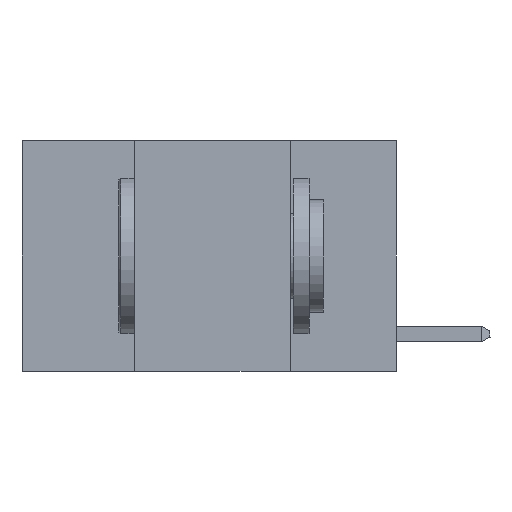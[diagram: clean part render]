
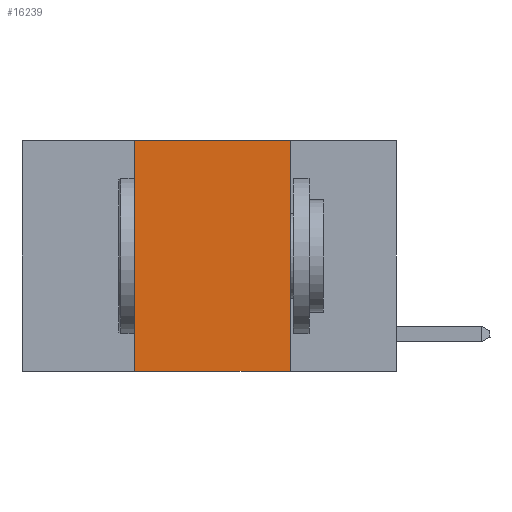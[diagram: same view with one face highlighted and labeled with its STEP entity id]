
A CAD part, left-side view. The second image highlights one B-rep face of the part: STEP entity #16239.
In plain terms, the highlighted planar face has unit normal (-1, 0, 0).
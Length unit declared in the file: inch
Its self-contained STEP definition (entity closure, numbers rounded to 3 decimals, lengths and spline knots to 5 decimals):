
#357 = VECTOR ( 'NONE', #3795, 39.37008 ) ;
#949 = VECTOR ( 'NONE', #24811, 39.37008 ) ;
#987 = DIRECTION ( 'NONE',  ( 0., -1., 0. ) ) ;
#1590 = CARTESIAN_POINT ( 'NONE',  ( 0., 0.17, 0. ) ) ;
#3172 = ORIENTED_EDGE ( 'NONE', *, *, #14653, .F. ) ;
#3487 = DIRECTION ( 'NONE',  ( 0., 0., 1. ) ) ;
#3795 = DIRECTION ( 'NONE',  ( 0., 0., -1. ) ) ;
#4456 = LINE ( 'NONE', #1590, #357 ) ;
#5049 = DIRECTION ( 'NONE',  ( 0., 0., -1. ) ) ;
#5169 = VERTEX_POINT ( 'NONE', #6675 ) ;
#6253 = LINE ( 'NONE', #16353, #23382 ) ;
#6347 = ORIENTED_EDGE ( 'NONE', *, *, #7418, .T. ) ;
#6675 = CARTESIAN_POINT ( 'NONE',  ( 0., 0.42, -0.37 ) ) ;
#6868 = AXIS2_PLACEMENT_3D ( 'NONE', #13619, #17924, #5049 ) ;
#7418 = EDGE_CURVE ( 'NONE', #5169, #11936, #12640, .T. ) ;
#7756 = CARTESIAN_POINT ( 'NONE',  ( 0., 0.42, 0. ) ) ;
#7850 = CARTESIAN_POINT ( 'NONE',  ( 0., 0.17, -0.37 ) ) ;
#8140 = VERTEX_POINT ( 'NONE', #7756 ) ;
#9190 = EDGE_LOOP ( 'NONE', ( #3172, #13420, #10382, #6347 ) ) ;
#10382 = ORIENTED_EDGE ( 'NONE', *, *, #13197, .F. ) ;
#11325 = VERTEX_POINT ( 'NONE', #14597 ) ;
#11936 = VERTEX_POINT ( 'NONE', #7850 ) ;
#12640 = LINE ( 'NONE', #13947, #24027 ) ;
#13197 = EDGE_CURVE ( 'NONE', #5169, #8140, #6253, .T. ) ;
#13420 = ORIENTED_EDGE ( 'NONE', *, *, #24505, .F. ) ;
#13619 = CARTESIAN_POINT ( 'NONE',  ( 0., 0.6, 0. ) ) ;
#13947 = CARTESIAN_POINT ( 'NONE',  ( 0., 0.6, -0.37 ) ) ;
#14166 = FACE_OUTER_BOUND ( 'NONE', #9190, .T. ) ;
#14597 = CARTESIAN_POINT ( 'NONE',  ( 0., 0.17, 0. ) ) ;
#14653 = EDGE_CURVE ( 'NONE', #11325, #11936, #4456, .T. ) ;
#15685 = PLANE ( 'NONE',  #6868 ) ;
#16239 = ADVANCED_FACE ( 'NONE', ( #14166 ), #15685, .F. ) ;
#16353 = CARTESIAN_POINT ( 'NONE',  ( 0., 0.42, 0. ) ) ;
#17924 = DIRECTION ( 'NONE',  ( 1., 0., 0. ) ) ;
#18168 = LINE ( 'NONE', #26842, #949 ) ;
#23382 = VECTOR ( 'NONE', #3487, 39.37008 ) ;
#24027 = VECTOR ( 'NONE', #987, 39.37008 ) ;
#24505 = EDGE_CURVE ( 'NONE', #8140, #11325, #18168, .T. ) ;
#24811 = DIRECTION ( 'NONE',  ( 0., -1., 0. ) ) ;
#26842 = CARTESIAN_POINT ( 'NONE',  ( 0., 0.6, 0. ) ) ;
